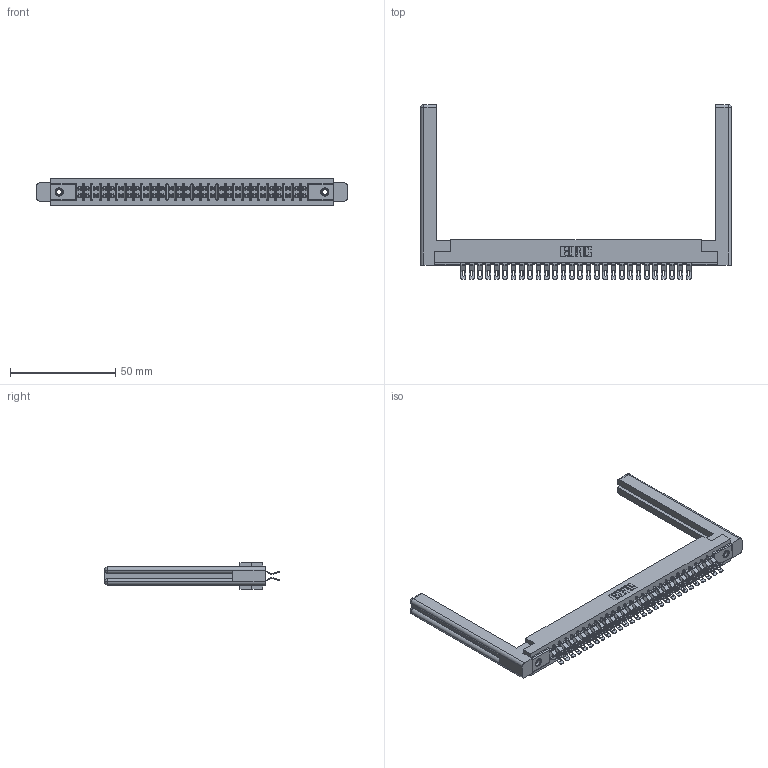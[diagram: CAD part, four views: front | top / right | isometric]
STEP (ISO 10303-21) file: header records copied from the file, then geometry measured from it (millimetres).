
FILE_DESCRIPTION (( 'STEP AP203' ), '1' );
FILE_NAME ('357-056-555-258.STEP', '2019-09-19T04:49:48', ( '' ), ( '' ), 'SwSTEP 2.0', 'SolidWorks 2016', '' );
FILE_SCHEMA (( 'CONFIG_CONTROL_DESIGN' ));
Length unit declared in the file: inch
Products named in the file (5): 307 Part_.156 Dia Mounting Holes; 307-220-058; 357-056-555-258; 307-290-001_555; 345-250-001_345-250-001-102
Assembly tree (61 placements, depth 2):
  357-056-555-258
    307 Part_.156 Dia Mounting Holes
    307-290-001_555  x56
    307-220-058  x2
    345-250-001_345-250-001-102  x2
Bounding box: 147.57 x 83.06 x 12.7 mm (x, y, z)
Volume: 22889.8 mm3; surface area: 24820.7 mm2
Topology: 61 solids, 61 shells, 3705 faces, 10813 edges, 7042 vertices
Faces by surface type: plane 2058, cylinder 1565, sphere 58, torus 12, cone 12
Entity records: 29796 total; most frequent: CARTESIAN_POINT 4903, ORIENTED_EDGE 4802, DIRECTION 4773, EDGE_CURVE 2401, LINE 1821, VECTOR 1821, VERTEX_POINT 1552, AXIS2_PLACEMENT_3D 1476
